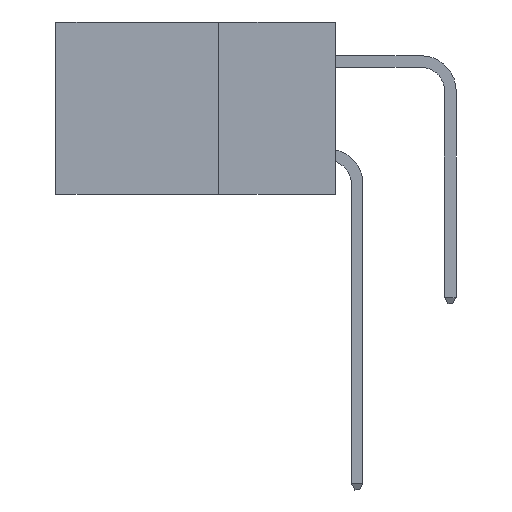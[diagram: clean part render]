
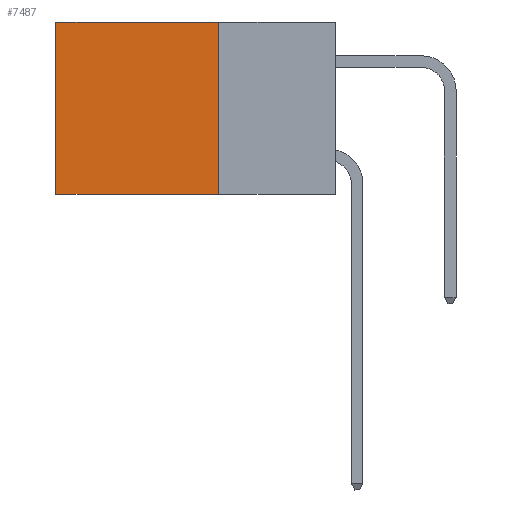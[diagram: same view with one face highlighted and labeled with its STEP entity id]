
A CAD part, left-side view. The second image highlights one B-rep face of the part: STEP entity #7487.
In plain terms, the highlighted planar face has unit normal (-1, 0, 0).
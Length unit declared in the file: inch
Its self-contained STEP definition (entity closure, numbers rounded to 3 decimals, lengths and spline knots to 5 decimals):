
#1669 = LINE ( 'NONE', #20782, #19978 ) ;
#2065 = VERTEX_POINT ( 'NONE', #18315 ) ;
#2192 = AXIS2_PLACEMENT_3D ( 'NONE', #13212, #2333, #14900 ) ;
#2333 = DIRECTION ( 'NONE',  ( 1., 0., 0. ) ) ;
#4430 = CARTESIAN_POINT ( 'NONE',  ( 0.2875, 0.25, 0. ) ) ;
#4510 = ORIENTED_EDGE ( 'NONE', *, *, #13707, .F. ) ;
#4847 = DIRECTION ( 'NONE',  ( 0., 1., 0. ) ) ;
#5587 = EDGE_LOOP ( 'NONE', ( #15508, #4510, #14421, #18081 ) ) ;
#6974 = DIRECTION ( 'NONE',  ( 0., 0., -1. ) ) ;
#7487 = ADVANCED_FACE ( 'NONE', ( #9984 ), #7847, .F. ) ;
#7783 = CARTESIAN_POINT ( 'NONE',  ( 0.2875, 0.25, -0.37 ) ) ;
#7847 = PLANE ( 'NONE',  #2192 ) ;
#8770 = LINE ( 'NONE', #10263, #16935 ) ;
#9329 = LINE ( 'NONE', #7783, #17974 ) ;
#9984 = FACE_OUTER_BOUND ( 'NONE', #5587, .T. ) ;
#10263 = CARTESIAN_POINT ( 'NONE',  ( 0.2875, 0.25, 0. ) ) ;
#10542 = CARTESIAN_POINT ( 'NONE',  ( 0.2875, 0.25, -0.37 ) ) ;
#12460 = VECTOR ( 'NONE', #18510, 39.37008 ) ;
#12725 = CARTESIAN_POINT ( 'NONE',  ( 0.2875, 0.25, 0. ) ) ;
#13212 = CARTESIAN_POINT ( 'NONE',  ( 0.2875, 0.25, 0. ) ) ;
#13325 = EDGE_CURVE ( 'NONE', #15417, #16962, #8770, .T. ) ;
#13707 = EDGE_CURVE ( 'NONE', #20068, #2065, #9329, .T. ) ;
#14421 = ORIENTED_EDGE ( 'NONE', *, *, #21004, .F. ) ;
#14900 = DIRECTION ( 'NONE',  ( 0., 0., -1. ) ) ;
#15417 = VERTEX_POINT ( 'NONE', #12725 ) ;
#15508 = ORIENTED_EDGE ( 'NONE', *, *, #19413, .T. ) ;
#16935 = VECTOR ( 'NONE', #4847, 39.37008 ) ;
#16962 = VERTEX_POINT ( 'NONE', #17345 ) ;
#17345 = CARTESIAN_POINT ( 'NONE',  ( 0.2875, 0.6, 0. ) ) ;
#17974 = VECTOR ( 'NONE', #21585, 39.37008 ) ;
#18081 = ORIENTED_EDGE ( 'NONE', *, *, #13325, .T. ) ;
#18315 = CARTESIAN_POINT ( 'NONE',  ( 0.2875, 0.6, -0.37 ) ) ;
#18510 = DIRECTION ( 'NONE',  ( 0., 0., -1. ) ) ;
#19413 = EDGE_CURVE ( 'NONE', #16962, #2065, #1669, .T. ) ;
#19978 = VECTOR ( 'NONE', #6974, 39.37008 ) ;
#20068 = VERTEX_POINT ( 'NONE', #10542 ) ;
#20782 = CARTESIAN_POINT ( 'NONE',  ( 0.2875, 0.6, 0. ) ) ;
#21004 = EDGE_CURVE ( 'NONE', #15417, #20068, #21998, .T. ) ;
#21585 = DIRECTION ( 'NONE',  ( 0., 1., 0. ) ) ;
#21998 = LINE ( 'NONE', #4430, #12460 ) ;
